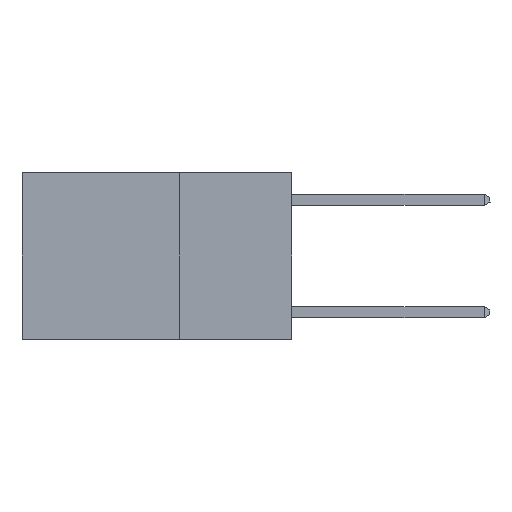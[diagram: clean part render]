
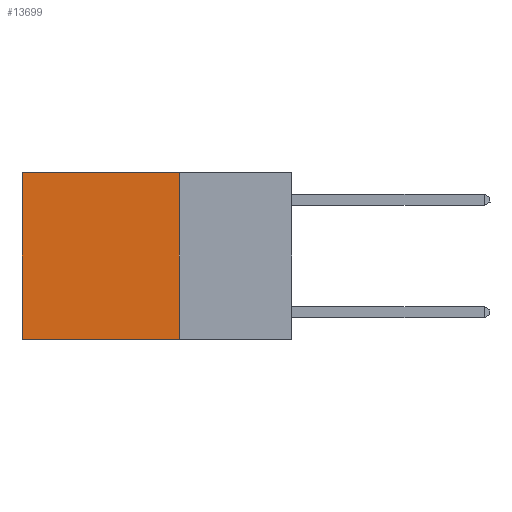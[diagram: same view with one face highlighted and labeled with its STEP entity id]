
A CAD part, left-side view. The second image highlights one B-rep face of the part: STEP entity #13699.
In plain terms, the highlighted planar face has unit normal (-1, 0, 0).
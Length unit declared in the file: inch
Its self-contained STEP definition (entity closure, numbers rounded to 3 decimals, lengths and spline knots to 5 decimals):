
#28 = CARTESIAN_POINT ( 'NONE',  ( 0.2625, 0.6, 0. ) ) ;
#479 = EDGE_CURVE ( 'NONE', #7840, #2947, #22021, .T. ) ;
#990 = VERTEX_POINT ( 'NONE', #16257 ) ;
#1800 = AXIS2_PLACEMENT_3D ( 'NONE', #14134, #5569, #10744 ) ;
#2947 = VERTEX_POINT ( 'NONE', #28 ) ;
#3569 = CARTESIAN_POINT ( 'NONE',  ( 0.2625, 0.25, -0.37 ) ) ;
#4362 = VERTEX_POINT ( 'NONE', #16704 ) ;
#4610 = DIRECTION ( 'NONE',  ( 0., 0., -1. ) ) ;
#5569 = DIRECTION ( 'NONE',  ( 1., 0., 0. ) ) ;
#5954 = VECTOR ( 'NONE', #19046, 39.37008 ) ;
#6064 = LINE ( 'NONE', #8309, #11733 ) ;
#6404 = ORIENTED_EDGE ( 'NONE', *, *, #17395, .F. ) ;
#7840 = VERTEX_POINT ( 'NONE', #17674 ) ;
#8309 = CARTESIAN_POINT ( 'NONE',  ( 0.2625, 0.6, 0. ) ) ;
#9682 = EDGE_CURVE ( 'NONE', #2947, #990, #6064, .T. ) ;
#10320 = EDGE_LOOP ( 'NONE', ( #15125, #6404, #14002, #18916 ) ) ;
#10744 = DIRECTION ( 'NONE',  ( 0., 0., -1. ) ) ;
#11584 = CARTESIAN_POINT ( 'NONE',  ( 0.2625, 0.25, 0. ) ) ;
#11733 = VECTOR ( 'NONE', #16858, 39.37008 ) ;
#12924 = VECTOR ( 'NONE', #4610, 39.37008 ) ;
#13699 = ADVANCED_FACE ( 'NONE', ( #16391 ), #21079, .F. ) ;
#14002 = ORIENTED_EDGE ( 'NONE', *, *, #21667, .F. ) ;
#14134 = CARTESIAN_POINT ( 'NONE',  ( 0.2625, 0.25, 0. ) ) ;
#14741 = DIRECTION ( 'NONE',  ( 0., 1., 0. ) ) ;
#14959 = CARTESIAN_POINT ( 'NONE',  ( 0.2625, 0.25, 0. ) ) ;
#15125 = ORIENTED_EDGE ( 'NONE', *, *, #9682, .T. ) ;
#15539 = VECTOR ( 'NONE', #14741, 39.37008 ) ;
#16176 = LINE ( 'NONE', #3569, #5954 ) ;
#16257 = CARTESIAN_POINT ( 'NONE',  ( 0.2625, 0.6, -0.37 ) ) ;
#16391 = FACE_OUTER_BOUND ( 'NONE', #10320, .T. ) ;
#16704 = CARTESIAN_POINT ( 'NONE',  ( 0.2625, 0.25, -0.37 ) ) ;
#16858 = DIRECTION ( 'NONE',  ( 0., 0., -1. ) ) ;
#17395 = EDGE_CURVE ( 'NONE', #4362, #990, #16176, .T. ) ;
#17674 = CARTESIAN_POINT ( 'NONE',  ( 0.2625, 0.25, 0. ) ) ;
#18916 = ORIENTED_EDGE ( 'NONE', *, *, #479, .T. ) ;
#19046 = DIRECTION ( 'NONE',  ( 0., 1., 0. ) ) ;
#21079 = PLANE ( 'NONE',  #1800 ) ;
#21544 = LINE ( 'NONE', #14959, #12924 ) ;
#21667 = EDGE_CURVE ( 'NONE', #7840, #4362, #21544, .T. ) ;
#22021 = LINE ( 'NONE', #11584, #15539 ) ;
